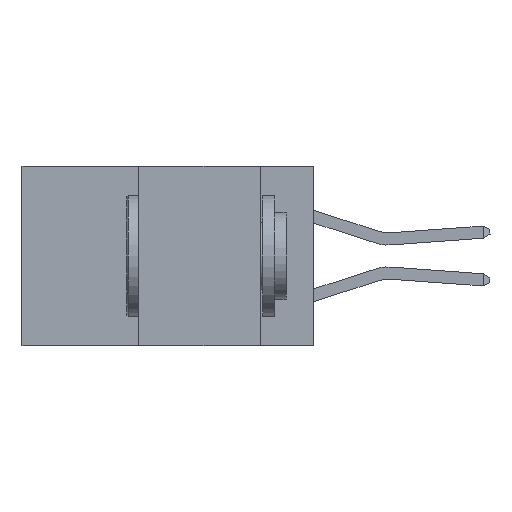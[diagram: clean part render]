
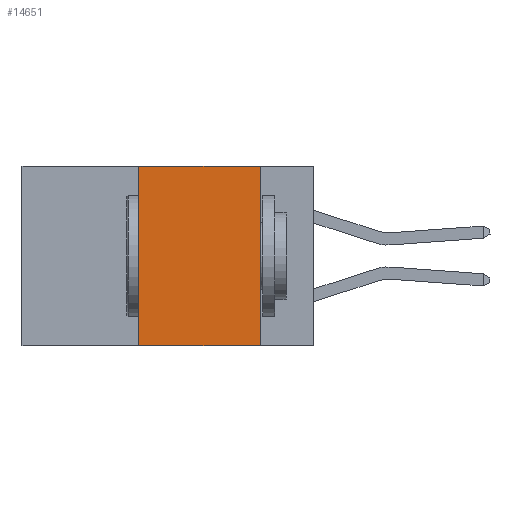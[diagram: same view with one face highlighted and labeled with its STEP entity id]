
A CAD part, left-side view. The second image highlights one B-rep face of the part: STEP entity #14651.
In plain terms, the highlighted planar face has unit normal (-1, 0, 0).
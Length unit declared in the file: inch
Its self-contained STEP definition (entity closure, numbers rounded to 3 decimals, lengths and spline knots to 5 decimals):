
#1546 = PLANE ( 'NONE',  #20148 ) ;
#1679 = DIRECTION ( 'NONE',  ( 0., 0., -1. ) ) ;
#2345 = LINE ( 'NONE', #14489, #33512 ) ;
#4989 = CARTESIAN_POINT ( 'NONE',  ( 0., 0.6, -0.37 ) ) ;
#5303 = VERTEX_POINT ( 'NONE', #38536 ) ;
#6454 = EDGE_LOOP ( 'NONE', ( #35567, #32341, #11103, #13941 ) ) ;
#8563 = DIRECTION ( 'NONE',  ( 0., -1., 0. ) ) ;
#9586 = EDGE_CURVE ( 'NONE', #12254, #25165, #15043, .T. ) ;
#11103 = ORIENTED_EDGE ( 'NONE', *, *, #24003, .F. ) ;
#11202 = FACE_OUTER_BOUND ( 'NONE', #6454, .T. ) ;
#11334 = VECTOR ( 'NONE', #26369, 39.37008 ) ;
#11392 = VECTOR ( 'NONE', #18801, 39.37008 ) ;
#12254 = VERTEX_POINT ( 'NONE', #17383 ) ;
#13941 = ORIENTED_EDGE ( 'NONE', *, *, #9586, .T. ) ;
#14082 = VECTOR ( 'NONE', #17029, 39.37008 ) ;
#14489 = CARTESIAN_POINT ( 'NONE',  ( 0., 0.6, 0. ) ) ;
#14651 = ADVANCED_FACE ( 'NONE', ( #11202 ), #1546, .F. ) ;
#15043 = LINE ( 'NONE', #4989, #14082 ) ;
#15738 = CARTESIAN_POINT ( 'NONE',  ( 0., 0.11, 0. ) ) ;
#16813 = CARTESIAN_POINT ( 'NONE',  ( 0., 0.6, 0. ) ) ;
#17029 = DIRECTION ( 'NONE',  ( 0., -1., 0. ) ) ;
#17383 = CARTESIAN_POINT ( 'NONE',  ( 0., 0.36, -0.37 ) ) ;
#17585 = CARTESIAN_POINT ( 'NONE',  ( 0., 0.11, -0.37 ) ) ;
#18801 = DIRECTION ( 'NONE',  ( 0., 0., -1. ) ) ;
#19883 = DIRECTION ( 'NONE',  ( 1., 0., 0. ) ) ;
#20148 = AXIS2_PLACEMENT_3D ( 'NONE', #16813, #19883, #1679 ) ;
#20379 = LINE ( 'NONE', #35207, #11334 ) ;
#24003 = EDGE_CURVE ( 'NONE', #12254, #5303, #20379, .T. ) ;
#25165 = VERTEX_POINT ( 'NONE', #17585 ) ;
#26369 = DIRECTION ( 'NONE',  ( 0., 0., 1. ) ) ;
#26863 = EDGE_CURVE ( 'NONE', #27118, #25165, #27503, .T. ) ;
#27118 = VERTEX_POINT ( 'NONE', #31916 ) ;
#27277 = EDGE_CURVE ( 'NONE', #5303, #27118, #2345, .T. ) ;
#27503 = LINE ( 'NONE', #15738, #11392 ) ;
#31916 = CARTESIAN_POINT ( 'NONE',  ( 0., 0.11, 0. ) ) ;
#32341 = ORIENTED_EDGE ( 'NONE', *, *, #27277, .F. ) ;
#33512 = VECTOR ( 'NONE', #8563, 39.37008 ) ;
#35207 = CARTESIAN_POINT ( 'NONE',  ( 0., 0.36, 0. ) ) ;
#35567 = ORIENTED_EDGE ( 'NONE', *, *, #26863, .F. ) ;
#38536 = CARTESIAN_POINT ( 'NONE',  ( 0., 0.36, 0. ) ) ;
